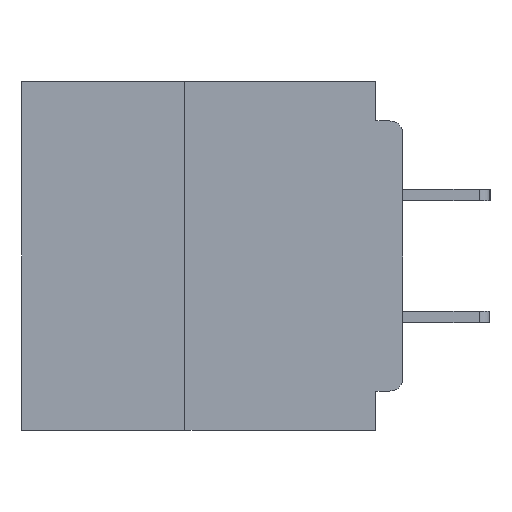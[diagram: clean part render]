
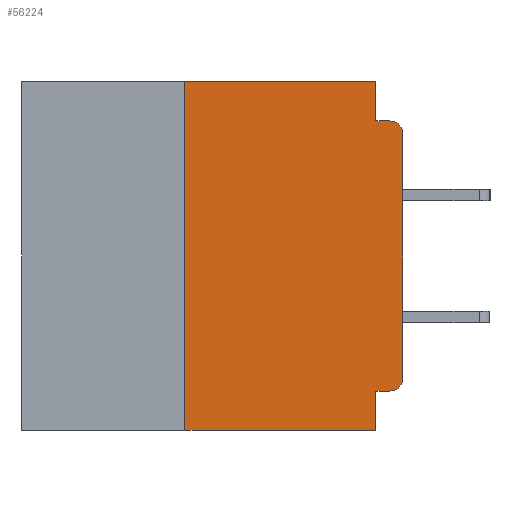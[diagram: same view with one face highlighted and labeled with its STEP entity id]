
A CAD part, left-side view. The second image highlights one B-rep face of the part: STEP entity #56224.
In plain terms, the highlighted planar face has unit normal (-1, 0, 0).
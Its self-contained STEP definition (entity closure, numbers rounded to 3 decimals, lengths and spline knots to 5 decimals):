
#358 = CARTESIAN_POINT ( 'NONE',  ( 0., 0.031, 0. ) ) ;
#1249 = VERTEX_POINT ( 'NONE', #46109 ) ;
#3117 = CARTESIAN_POINT ( 'NONE',  ( 0., 0.031, -0.045 ) ) ;
#3410 = EDGE_CURVE ( 'NONE', #4183, #54409, #63756, .T. ) ;
#3539 = VERTEX_POINT ( 'NONE', #32500 ) ;
#3722 = ORIENTED_EDGE ( 'NONE', *, *, #40567, .F. ) ;
#3760 = CARTESIAN_POINT ( 'NONE',  ( 0., 0.437, 0. ) ) ;
#3848 = VERTEX_POINT ( 'NONE', #5616 ) ;
#4183 = VERTEX_POINT ( 'NONE', #62560 ) ;
#5325 = DIRECTION ( 'NONE',  ( 0., 0., -1. ) ) ;
#5616 = CARTESIAN_POINT ( 'NONE',  ( 0., 0.031, -0.355 ) ) ;
#6144 = ORIENTED_EDGE ( 'NONE', *, *, #40967, .F. ) ;
#8761 = DIRECTION ( 'NONE',  ( 0., 0., -1. ) ) ;
#9203 = VECTOR ( 'NONE', #43564, 39.37008 ) ;
#9832 = LINE ( 'NONE', #18940, #33000 ) ;
#10260 = CARTESIAN_POINT ( 'NONE',  ( 0., 0.25, -0.4 ) ) ;
#11059 = VECTOR ( 'NONE', #30603, 39.37008 ) ;
#13950 = DIRECTION ( 'NONE',  ( 0., -1., 0. ) ) ;
#15277 = EDGE_CURVE ( 'NONE', #51838, #3539, #50023, .T. ) ;
#15339 = VERTEX_POINT ( 'NONE', #43985 ) ;
#15821 = ORIENTED_EDGE ( 'NONE', *, *, #55965, .T. ) ;
#18940 = CARTESIAN_POINT ( 'NONE',  ( 0., 0., -0.045 ) ) ;
#19956 = CARTESIAN_POINT ( 'NONE',  ( 0., 0.015, -0.045 ) ) ;
#21312 = LINE ( 'NONE', #358, #41366 ) ;
#21325 = CARTESIAN_POINT ( 'NONE',  ( 0., 0., 0. ) ) ;
#21697 = EDGE_CURVE ( 'NONE', #3848, #3539, #26918, .T. ) ;
#22307 = ORIENTED_EDGE ( 'NONE', *, *, #48400, .T. ) ;
#23261 = CARTESIAN_POINT ( 'NONE',  ( 0., 0.031, -0.4 ) ) ;
#23424 = PLANE ( 'NONE',  #28163 ) ;
#24057 = VERTEX_POINT ( 'NONE', #3117 ) ;
#25215 = AXIS2_PLACEMENT_3D ( 'NONE', #48328, #48281, #48274 ) ;
#26051 = CARTESIAN_POINT ( 'NONE',  ( 0., 0.015, -0.06 ) ) ;
#26251 = DIRECTION ( 'NONE',  ( 0., 0., 1. ) ) ;
#26586 = ORIENTED_EDGE ( 'NONE', *, *, #15277, .T. ) ;
#26918 = LINE ( 'NONE', #23261, #36970 ) ;
#28163 = AXIS2_PLACEMENT_3D ( 'NONE', #3760, #38353, #8761 ) ;
#28790 = VECTOR ( 'NONE', #59120, 39.37008 ) ;
#30379 = CARTESIAN_POINT ( 'NONE',  ( 0., 0.031, 0. ) ) ;
#30603 = DIRECTION ( 'NONE',  ( 0., -1., 0. ) ) ;
#31041 = DIRECTION ( 'NONE',  ( 0., 0., -1. ) ) ;
#32500 = CARTESIAN_POINT ( 'NONE',  ( 0., 0.031, -0.4 ) ) ;
#32940 = CARTESIAN_POINT ( 'NONE',  ( 0., 0., -0.34 ) ) ;
#33000 = VECTOR ( 'NONE', #13950, 39.37008 ) ;
#33510 = EDGE_CURVE ( 'NONE', #35465, #24057, #21312, .T. ) ;
#35465 = VERTEX_POINT ( 'NONE', #30379 ) ;
#35486 = AXIS2_PLACEMENT_3D ( 'NONE', #26051, #60427, #31041 ) ;
#36970 = VECTOR ( 'NONE', #52902, 39.37008 ) ;
#37571 = LINE ( 'NONE', #21325, #49032 ) ;
#38292 = LINE ( 'NONE', #56049, #51287 ) ;
#38353 = DIRECTION ( 'NONE',  ( 1., 0., 0. ) ) ;
#38672 = CARTESIAN_POINT ( 'NONE',  ( 0., 0.437, -0.4 ) ) ;
#39469 = EDGE_CURVE ( 'NONE', #51838, #15339, #38292, .T. ) ;
#40567 = EDGE_CURVE ( 'NONE', #15339, #35465, #50353, .T. ) ;
#40967 = EDGE_CURVE ( 'NONE', #4183, #3848, #43421, .T. ) ;
#41366 = VECTOR ( 'NONE', #5325, 39.37008 ) ;
#41934 = ORIENTED_EDGE ( 'NONE', *, *, #3410, .T. ) ;
#42942 = VERTEX_POINT ( 'NONE', #19956 ) ;
#43421 = LINE ( 'NONE', #58909, #28790 ) ;
#43564 = DIRECTION ( 'NONE',  ( 0., -1., 0. ) ) ;
#43985 = CARTESIAN_POINT ( 'NONE',  ( 0., 0.25, 0. ) ) ;
#44079 = ORIENTED_EDGE ( 'NONE', *, *, #21697, .F. ) ;
#45116 = ORIENTED_EDGE ( 'NONE', *, *, #39469, .F. ) ;
#45208 = CARTESIAN_POINT ( 'NONE',  ( 0., 0.437, 0. ) ) ;
#46109 = CARTESIAN_POINT ( 'NONE',  ( 0., 0., -0.06 ) ) ;
#46219 = DIRECTION ( 'NONE',  ( 0., 0., 1. ) ) ;
#47085 = EDGE_LOOP ( 'NONE', ( #15821, #22307, #47858, #49855, #3722, #45116, #26586, #44079, #6144, #41934 ) ) ;
#47858 = ORIENTED_EDGE ( 'NONE', *, *, #61008, .F. ) ;
#48228 = FACE_OUTER_BOUND ( 'NONE', #47085, .T. ) ;
#48274 = DIRECTION ( 'NONE',  ( 0., 0., -1. ) ) ;
#48281 = DIRECTION ( 'NONE',  ( -1., 0., 0. ) ) ;
#48328 = CARTESIAN_POINT ( 'NONE',  ( 0., 0.015, -0.34 ) ) ;
#48400 = EDGE_CURVE ( 'NONE', #1249, #42942, #53393, .T. ) ;
#49032 = VECTOR ( 'NONE', #26251, 39.37008 ) ;
#49855 = ORIENTED_EDGE ( 'NONE', *, *, #33510, .F. ) ;
#50023 = LINE ( 'NONE', #38672, #9203 ) ;
#50353 = LINE ( 'NONE', #45208, #11059 ) ;
#51287 = VECTOR ( 'NONE', #46219, 39.37008 ) ;
#51838 = VERTEX_POINT ( 'NONE', #10260 ) ;
#52902 = DIRECTION ( 'NONE',  ( 0., 0., -1. ) ) ;
#53393 = CIRCLE ( 'NONE', #35486, 0.015 ) ;
#54409 = VERTEX_POINT ( 'NONE', #32940 ) ;
#55965 = EDGE_CURVE ( 'NONE', #54409, #1249, #37571, .T. ) ;
#56049 = CARTESIAN_POINT ( 'NONE',  ( 0., 0.25, -0.4 ) ) ;
#56224 = ADVANCED_FACE ( 'NONE', ( #48228 ), #23424, .F. ) ;
#58909 = CARTESIAN_POINT ( 'NONE',  ( 0., 0., -0.355 ) ) ;
#59120 = DIRECTION ( 'NONE',  ( 0., 1., 0. ) ) ;
#60427 = DIRECTION ( 'NONE',  ( -1., 0., 0. ) ) ;
#61008 = EDGE_CURVE ( 'NONE', #24057, #42942, #9832, .T. ) ;
#62560 = CARTESIAN_POINT ( 'NONE',  ( 0., 0.015, -0.355 ) ) ;
#63756 = CIRCLE ( 'NONE', #25215, 0.015 ) ;
